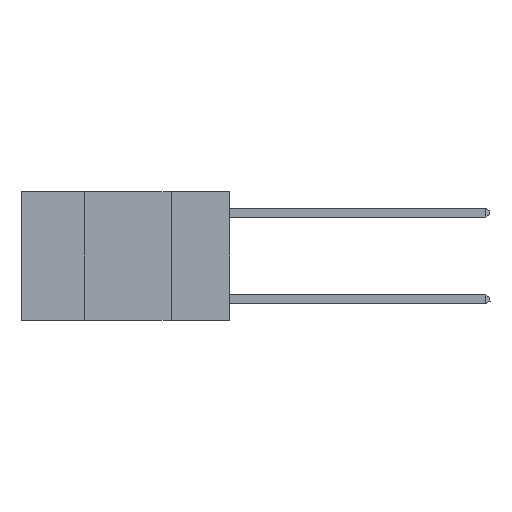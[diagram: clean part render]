
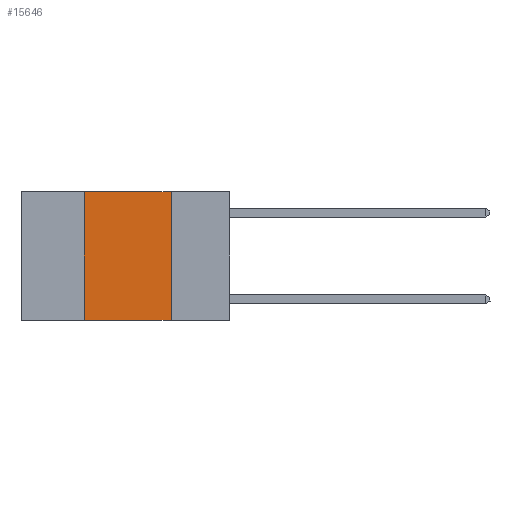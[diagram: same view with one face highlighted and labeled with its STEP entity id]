
A CAD part, left-side view. The second image highlights one B-rep face of the part: STEP entity #15646.
In plain terms, the highlighted planar face has unit normal (-1, 0, 0).
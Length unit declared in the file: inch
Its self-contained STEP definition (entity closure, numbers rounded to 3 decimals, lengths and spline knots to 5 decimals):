
#13 = CARTESIAN_POINT ( 'NONE',  ( 0., 0.17, 0. ) ) ;
#638 = CARTESIAN_POINT ( 'NONE',  ( 0., 0.6, 0. ) ) ;
#846 = EDGE_CURVE ( 'NONE', #2272, #15225, #15461, .T. ) ;
#1330 = CARTESIAN_POINT ( 'NONE',  ( 0., 0.6, 0. ) ) ;
#1383 = EDGE_CURVE ( 'NONE', #3994, #15225, #13018, .T. ) ;
#1930 = DIRECTION ( 'NONE',  ( 0., 0., -1. ) ) ;
#2272 = VERTEX_POINT ( 'NONE', #13 ) ;
#2628 = LINE ( 'NONE', #1330, #12098 ) ;
#3419 = CARTESIAN_POINT ( 'NONE',  ( 0., 0.42, 0. ) ) ;
#3729 = DIRECTION ( 'NONE',  ( 0., -1., 0. ) ) ;
#3994 = VERTEX_POINT ( 'NONE', #6537 ) ;
#4486 = DIRECTION ( 'NONE',  ( 0., 0., 1. ) ) ;
#5316 = ORIENTED_EDGE ( 'NONE', *, *, #1383, .T. ) ;
#5792 = CARTESIAN_POINT ( 'NONE',  ( 0., 0.17, 0. ) ) ;
#6117 = AXIS2_PLACEMENT_3D ( 'NONE', #638, #9660, #1930 ) ;
#6150 = VECTOR ( 'NONE', #3729, 39.37008 ) ;
#6499 = EDGE_CURVE ( 'NONE', #3994, #12658, #8493, .T. ) ;
#6537 = CARTESIAN_POINT ( 'NONE',  ( 0., 0.42, -0.37 ) ) ;
#7519 = CARTESIAN_POINT ( 'NONE',  ( 0., 0.17, -0.37 ) ) ;
#7742 = DIRECTION ( 'NONE',  ( 0., -1., 0. ) ) ;
#8065 = ORIENTED_EDGE ( 'NONE', *, *, #846, .F. ) ;
#8493 = LINE ( 'NONE', #12187, #16182 ) ;
#9028 = FACE_OUTER_BOUND ( 'NONE', #13713, .T. ) ;
#9660 = DIRECTION ( 'NONE',  ( 1., 0., 0. ) ) ;
#10872 = PLANE ( 'NONE',  #6117 ) ;
#11318 = ORIENTED_EDGE ( 'NONE', *, *, #14229, .F. ) ;
#12098 = VECTOR ( 'NONE', #7742, 39.37008 ) ;
#12187 = CARTESIAN_POINT ( 'NONE',  ( 0., 0.42, 0. ) ) ;
#12476 = CARTESIAN_POINT ( 'NONE',  ( 0., 0.6, -0.37 ) ) ;
#12658 = VERTEX_POINT ( 'NONE', #3419 ) ;
#13018 = LINE ( 'NONE', #12476, #6150 ) ;
#13713 = EDGE_LOOP ( 'NONE', ( #8065, #11318, #14332, #5316 ) ) ;
#14229 = EDGE_CURVE ( 'NONE', #12658, #2272, #2628, .T. ) ;
#14332 = ORIENTED_EDGE ( 'NONE', *, *, #6499, .F. ) ;
#14759 = DIRECTION ( 'NONE',  ( 0., 0., -1. ) ) ;
#15052 = VECTOR ( 'NONE', #14759, 39.37008 ) ;
#15225 = VERTEX_POINT ( 'NONE', #7519 ) ;
#15461 = LINE ( 'NONE', #5792, #15052 ) ;
#15646 = ADVANCED_FACE ( 'NONE', ( #9028 ), #10872, .F. ) ;
#16182 = VECTOR ( 'NONE', #4486, 39.37008 ) ;
